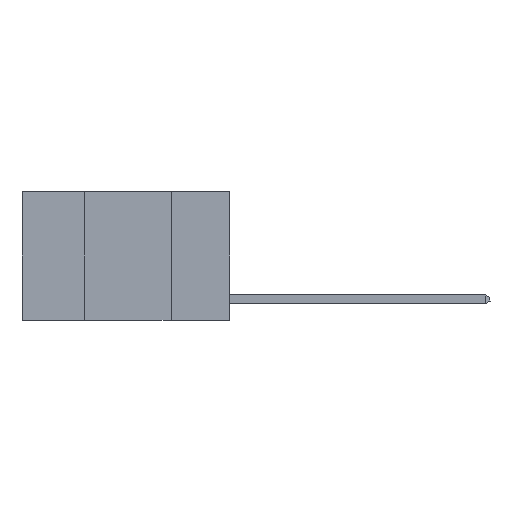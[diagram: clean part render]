
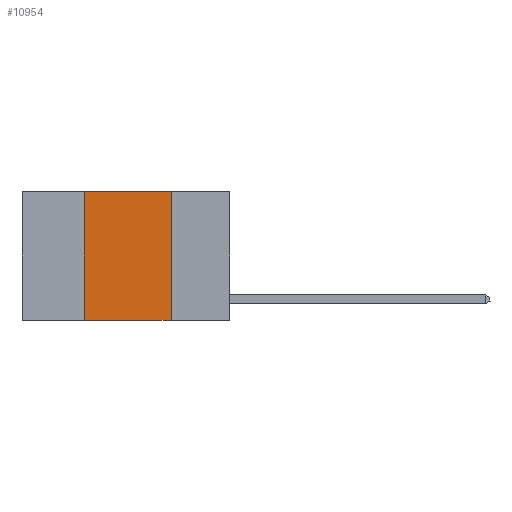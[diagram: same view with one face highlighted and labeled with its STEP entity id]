
A CAD part, left-side view. The second image highlights one B-rep face of the part: STEP entity #10954.
In plain terms, the highlighted planar face has unit normal (-1, 0, 0).
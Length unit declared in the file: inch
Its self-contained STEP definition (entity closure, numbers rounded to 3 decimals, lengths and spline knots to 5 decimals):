
#88 = LINE ( 'NONE', #9580, #16970 ) ;
#116 = EDGE_CURVE ( 'NONE', #5360, #13338, #10356, .T. ) ;
#1735 = LINE ( 'NONE', #6803, #16076 ) ;
#2359 = VERTEX_POINT ( 'NONE', #5521 ) ;
#2776 = PLANE ( 'NONE',  #8551 ) ;
#3204 = VERTEX_POINT ( 'NONE', #12597 ) ;
#4358 = ORIENTED_EDGE ( 'NONE', *, *, #18731, .F. ) ;
#5360 = VERTEX_POINT ( 'NONE', #9568 ) ;
#5521 = CARTESIAN_POINT ( 'NONE',  ( 0., 0.42, 0. ) ) ;
#5767 = DIRECTION ( 'NONE',  ( 0., 0., -1. ) ) ;
#5980 = CARTESIAN_POINT ( 'NONE',  ( 0., 0.17, 0. ) ) ;
#6803 = CARTESIAN_POINT ( 'NONE',  ( 0., 0.6, -0.37 ) ) ;
#6956 = EDGE_CURVE ( 'NONE', #3204, #13338, #1735, .T. ) ;
#8076 = CARTESIAN_POINT ( 'NONE',  ( 0., 0.17, -0.37 ) ) ;
#8551 = AXIS2_PLACEMENT_3D ( 'NONE', #16284, #19354, #5767 ) ;
#9568 = CARTESIAN_POINT ( 'NONE',  ( 0., 0.17, 0. ) ) ;
#9580 = CARTESIAN_POINT ( 'NONE',  ( 0., 0.42, 0. ) ) ;
#9877 = CARTESIAN_POINT ( 'NONE',  ( 0., 0.6, 0. ) ) ;
#10356 = LINE ( 'NONE', #5980, #10828 ) ;
#10489 = VECTOR ( 'NONE', #11055, 39.37008 ) ;
#10828 = VECTOR ( 'NONE', #12061, 39.37008 ) ;
#10954 = ADVANCED_FACE ( 'NONE', ( #11232 ), #2776, .F. ) ;
#10970 = DIRECTION ( 'NONE',  ( 0., 0., 1. ) ) ;
#11026 = ORIENTED_EDGE ( 'NONE', *, *, #116, .F. ) ;
#11055 = DIRECTION ( 'NONE',  ( 0., -1., 0. ) ) ;
#11232 = FACE_OUTER_BOUND ( 'NONE', #13930, .T. ) ;
#11667 = ORIENTED_EDGE ( 'NONE', *, *, #12249, .F. ) ;
#12061 = DIRECTION ( 'NONE',  ( 0., 0., -1. ) ) ;
#12249 = EDGE_CURVE ( 'NONE', #2359, #5360, #18186, .T. ) ;
#12597 = CARTESIAN_POINT ( 'NONE',  ( 0., 0.42, -0.37 ) ) ;
#13122 = ORIENTED_EDGE ( 'NONE', *, *, #6956, .T. ) ;
#13338 = VERTEX_POINT ( 'NONE', #8076 ) ;
#13930 = EDGE_LOOP ( 'NONE', ( #11026, #11667, #4358, #13122 ) ) ;
#15968 = DIRECTION ( 'NONE',  ( 0., -1., 0. ) ) ;
#16076 = VECTOR ( 'NONE', #15968, 39.37008 ) ;
#16284 = CARTESIAN_POINT ( 'NONE',  ( 0., 0.6, 0. ) ) ;
#16970 = VECTOR ( 'NONE', #10970, 39.37008 ) ;
#18186 = LINE ( 'NONE', #9877, #10489 ) ;
#18731 = EDGE_CURVE ( 'NONE', #3204, #2359, #88, .T. ) ;
#19354 = DIRECTION ( 'NONE',  ( 1., 0., 0. ) ) ;
